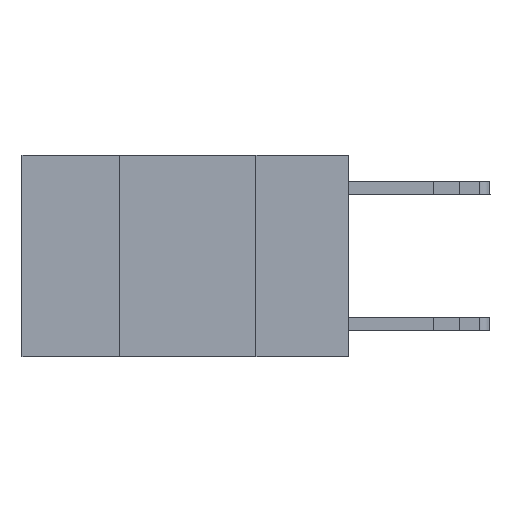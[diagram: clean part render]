
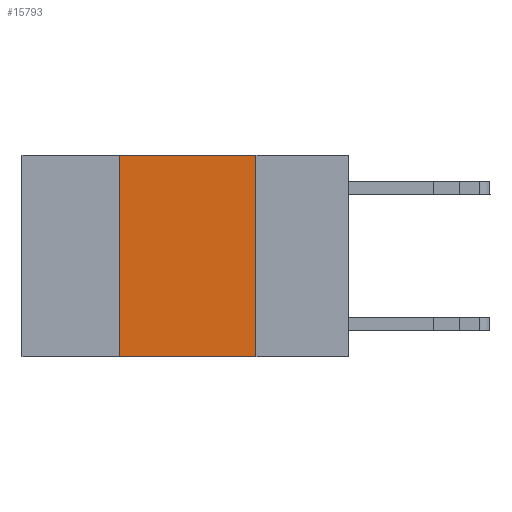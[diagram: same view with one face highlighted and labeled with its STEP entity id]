
A CAD part, left-side view. The second image highlights one B-rep face of the part: STEP entity #15793.
In plain terms, the highlighted planar face has unit normal (-1, 0, 0).
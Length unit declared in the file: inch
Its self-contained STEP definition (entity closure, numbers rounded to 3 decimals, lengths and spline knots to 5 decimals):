
#128 = VECTOR ( 'NONE', #20355, 39.37008 ) ;
#182 = LINE ( 'NONE', #4371, #128 ) ;
#3888 = ORIENTED_EDGE ( 'NONE', *, *, #7780, .F. ) ;
#4371 = CARTESIAN_POINT ( 'NONE',  ( 0., 0.42, 0. ) ) ;
#5120 = EDGE_CURVE ( 'NONE', #17492, #15912, #11100, .T. ) ;
#7020 = DIRECTION ( 'NONE',  ( 0., -1., 0. ) ) ;
#7061 = AXIS2_PLACEMENT_3D ( 'NONE', #7740, #11849, #25420 ) ;
#7330 = CARTESIAN_POINT ( 'NONE',  ( 0., 0.6, -0.37 ) ) ;
#7740 = CARTESIAN_POINT ( 'NONE',  ( 0., 0.6, 0. ) ) ;
#7780 = EDGE_CURVE ( 'NONE', #15912, #9807, #19911, .T. ) ;
#7940 = ORIENTED_EDGE ( 'NONE', *, *, #5120, .F. ) ;
#9146 = EDGE_CURVE ( 'NONE', #22324, #9807, #25222, .T. ) ;
#9807 = VERTEX_POINT ( 'NONE', #12430 ) ;
#10644 = ORIENTED_EDGE ( 'NONE', *, *, #18897, .F. ) ;
#10879 = VECTOR ( 'NONE', #14922, 39.37008 ) ;
#11100 = LINE ( 'NONE', #14832, #10879 ) ;
#11849 = DIRECTION ( 'NONE',  ( 1., 0., 0. ) ) ;
#12176 = CARTESIAN_POINT ( 'NONE',  ( 0., 0.17, 0. ) ) ;
#12430 = CARTESIAN_POINT ( 'NONE',  ( 0., 0.17, -0.37 ) ) ;
#14139 = CARTESIAN_POINT ( 'NONE',  ( 0., 0.17, 0. ) ) ;
#14832 = CARTESIAN_POINT ( 'NONE',  ( 0., 0.6, 0. ) ) ;
#14922 = DIRECTION ( 'NONE',  ( 0., -1., 0. ) ) ;
#15480 = ORIENTED_EDGE ( 'NONE', *, *, #9146, .T. ) ;
#15793 = ADVANCED_FACE ( 'NONE', ( #23442 ), #15802, .F. ) ;
#15802 = PLANE ( 'NONE',  #7061 ) ;
#15912 = VERTEX_POINT ( 'NONE', #14139 ) ;
#17492 = VERTEX_POINT ( 'NONE', #22586 ) ;
#18349 = VECTOR ( 'NONE', #22966, 39.37008 ) ;
#18897 = EDGE_CURVE ( 'NONE', #22324, #17492, #182, .T. ) ;
#19911 = LINE ( 'NONE', #12176, #18349 ) ;
#20355 = DIRECTION ( 'NONE',  ( 0., 0., 1. ) ) ;
#21670 = EDGE_LOOP ( 'NONE', ( #3888, #7940, #10644, #15480 ) ) ;
#22324 = VERTEX_POINT ( 'NONE', #22492 ) ;
#22492 = CARTESIAN_POINT ( 'NONE',  ( 0., 0.42, -0.37 ) ) ;
#22586 = CARTESIAN_POINT ( 'NONE',  ( 0., 0.42, 0. ) ) ;
#22966 = DIRECTION ( 'NONE',  ( 0., 0., -1. ) ) ;
#23442 = FACE_OUTER_BOUND ( 'NONE', #21670, .T. ) ;
#24820 = VECTOR ( 'NONE', #7020, 39.37008 ) ;
#25222 = LINE ( 'NONE', #7330, #24820 ) ;
#25420 = DIRECTION ( 'NONE',  ( 0., 0., -1. ) ) ;
